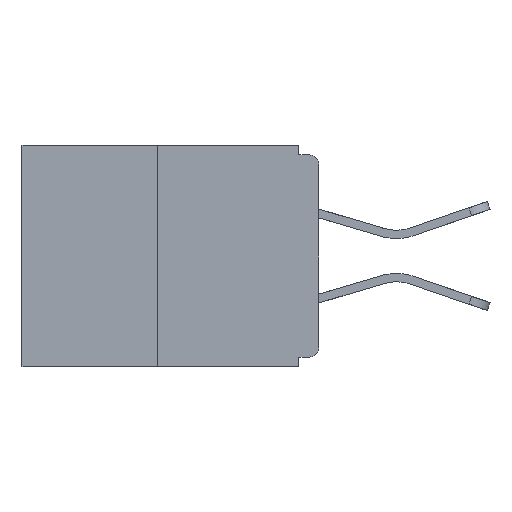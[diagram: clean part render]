
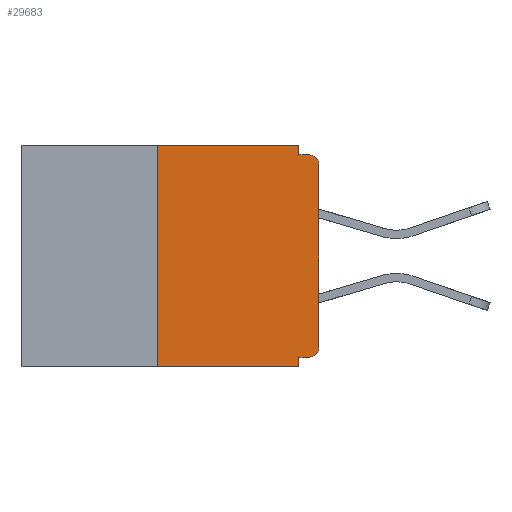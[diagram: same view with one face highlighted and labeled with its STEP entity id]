
A CAD part, left-side view. The second image highlights one B-rep face of the part: STEP entity #29683.
In plain terms, the highlighted planar face has unit normal (-1, 0, 0).
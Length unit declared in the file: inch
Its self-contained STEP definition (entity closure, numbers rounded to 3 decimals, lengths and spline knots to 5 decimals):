
#731 = VECTOR ( 'NONE', #14783, 39.37008 ) ;
#1760 = VECTOR ( 'NONE', #10039, 39.37008 ) ;
#2047 = CIRCLE ( 'NONE', #9286, 0.015 ) ;
#2706 = ORIENTED_EDGE ( 'NONE', *, *, #6965, .F. ) ;
#2714 = ORIENTED_EDGE ( 'NONE', *, *, #26949, .F. ) ;
#3550 = CARTESIAN_POINT ( 'NONE',  ( 0., 0.015, -0.328 ) ) ;
#3679 = VERTEX_POINT ( 'NONE', #21947 ) ;
#3745 = CARTESIAN_POINT ( 'NONE',  ( 0., 0.015, -0.03 ) ) ;
#3855 = DIRECTION ( 'NONE',  ( 0., 0., -1. ) ) ;
#4433 = LINE ( 'NONE', #21259, #26086 ) ;
#4735 = FACE_OUTER_BOUND ( 'NONE', #29015, .T. ) ;
#5065 = ORIENTED_EDGE ( 'NONE', *, *, #28277, .T. ) ;
#5213 = CARTESIAN_POINT ( 'NONE',  ( 0., 0., 0. ) ) ;
#5677 = DIRECTION ( 'NONE',  ( -1., 0., 0. ) ) ;
#5901 = ORIENTED_EDGE ( 'NONE', *, *, #29616, .T. ) ;
#6394 = CARTESIAN_POINT ( 'NONE',  ( 0., 0.031, -0.015 ) ) ;
#6450 = DIRECTION ( 'NONE',  ( 0., 0., -1. ) ) ;
#6664 = CARTESIAN_POINT ( 'NONE',  ( 0., 0., -0.03 ) ) ;
#6965 = EDGE_CURVE ( 'NONE', #22255, #7454, #16489, .T. ) ;
#7068 = VERTEX_POINT ( 'NONE', #9651 ) ;
#7406 = CARTESIAN_POINT ( 'NONE',  ( 0., 0., -0.328 ) ) ;
#7454 = VERTEX_POINT ( 'NONE', #6394 ) ;
#7911 = VERTEX_POINT ( 'NONE', #6664 ) ;
#8894 = CARTESIAN_POINT ( 'NONE',  ( 0., 0.46, -0.343 ) ) ;
#9176 = VECTOR ( 'NONE', #12169, 39.37008 ) ;
#9286 = AXIS2_PLACEMENT_3D ( 'NONE', #3745, #18150, #3855 ) ;
#9651 = CARTESIAN_POINT ( 'NONE',  ( 0., 0., -0.313 ) ) ;
#10039 = DIRECTION ( 'NONE',  ( 0., 0., 1. ) ) ;
#10164 = VECTOR ( 'NONE', #16411, 39.37008 ) ;
#10218 = VERTEX_POINT ( 'NONE', #18093 ) ;
#10365 = CARTESIAN_POINT ( 'NONE',  ( 0., 0.015, -0.313 ) ) ;
#10588 = LINE ( 'NONE', #8894, #20694 ) ;
#10612 = DIRECTION ( 'NONE',  ( 0., 0., -1. ) ) ;
#12142 = ORIENTED_EDGE ( 'NONE', *, *, #27635, .F. ) ;
#12169 = DIRECTION ( 'NONE',  ( 0., 1., 0. ) ) ;
#13222 = CARTESIAN_POINT ( 'NONE',  ( 0., 0.031, -0.343 ) ) ;
#13822 = EDGE_CURVE ( 'NONE', #26939, #7068, #23405, .T. ) ;
#14033 = CARTESIAN_POINT ( 'NONE',  ( 0., 0.031, -0.328 ) ) ;
#14430 = LINE ( 'NONE', #5213, #1760 ) ;
#14516 = VERTEX_POINT ( 'NONE', #14033 ) ;
#14783 = DIRECTION ( 'NONE',  ( 0., -1., 0. ) ) ;
#15462 = AXIS2_PLACEMENT_3D ( 'NONE', #10365, #5677, #22162 ) ;
#16190 = EDGE_CURVE ( 'NONE', #7911, #3679, #2047, .T. ) ;
#16411 = DIRECTION ( 'NONE',  ( 0., 0., -1. ) ) ;
#16489 = LINE ( 'NONE', #16616, #10164 ) ;
#16616 = CARTESIAN_POINT ( 'NONE',  ( 0., 0.031, 0. ) ) ;
#17787 = VECTOR ( 'NONE', #10612, 39.37008 ) ;
#18093 = CARTESIAN_POINT ( 'NONE',  ( 0., 0.25, 0. ) ) ;
#18150 = DIRECTION ( 'NONE',  ( -1., 0., 0. ) ) ;
#18201 = ORIENTED_EDGE ( 'NONE', *, *, #24262, .F. ) ;
#18871 = CARTESIAN_POINT ( 'NONE',  ( 0., 0.25, -0.343 ) ) ;
#18930 = ORIENTED_EDGE ( 'NONE', *, *, #16190, .T. ) ;
#18976 = DIRECTION ( 'NONE',  ( 0., -1., 0. ) ) ;
#19293 = VERTEX_POINT ( 'NONE', #13222 ) ;
#19565 = ORIENTED_EDGE ( 'NONE', *, *, #13822, .T. ) ;
#20343 = CARTESIAN_POINT ( 'NONE',  ( 0., 0.031, -0.343 ) ) ;
#20694 = VECTOR ( 'NONE', #21111, 39.37008 ) ;
#21021 = EDGE_CURVE ( 'NONE', #14516, #19293, #22283, .T. ) ;
#21111 = DIRECTION ( 'NONE',  ( 0., -1., 0. ) ) ;
#21259 = CARTESIAN_POINT ( 'NONE',  ( 0., 0.25, 0. ) ) ;
#21947 = CARTESIAN_POINT ( 'NONE',  ( 0., 0.015, -0.015 ) ) ;
#22109 = CARTESIAN_POINT ( 'NONE',  ( 0., 0., -0.015 ) ) ;
#22162 = DIRECTION ( 'NONE',  ( 0., 0., -1. ) ) ;
#22255 = VERTEX_POINT ( 'NONE', #22966 ) ;
#22283 = LINE ( 'NONE', #20343, #17787 ) ;
#22966 = CARTESIAN_POINT ( 'NONE',  ( 0., 0.031, 0. ) ) ;
#22975 = PLANE ( 'NONE',  #29574 ) ;
#23405 = CIRCLE ( 'NONE', #15462, 0.015 ) ;
#23716 = VECTOR ( 'NONE', #18976, 39.37008 ) ;
#24262 = EDGE_CURVE ( 'NONE', #7454, #3679, #26142, .T. ) ;
#24696 = EDGE_CURVE ( 'NONE', #27689, #10218, #4433, .T. ) ;
#25203 = LINE ( 'NONE', #30383, #23716 ) ;
#25345 = CARTESIAN_POINT ( 'NONE',  ( 0., 0.46, 0. ) ) ;
#25649 = DIRECTION ( 'NONE',  ( 1., 0., 0. ) ) ;
#26086 = VECTOR ( 'NONE', #28238, 39.37008 ) ;
#26142 = LINE ( 'NONE', #22109, #731 ) ;
#26939 = VERTEX_POINT ( 'NONE', #3550 ) ;
#26949 = EDGE_CURVE ( 'NONE', #26939, #14516, #28229, .T. ) ;
#27635 = EDGE_CURVE ( 'NONE', #10218, #22255, #25203, .T. ) ;
#27689 = VERTEX_POINT ( 'NONE', #18871 ) ;
#28229 = LINE ( 'NONE', #7406, #9176 ) ;
#28238 = DIRECTION ( 'NONE',  ( 0., 0., 1. ) ) ;
#28277 = EDGE_CURVE ( 'NONE', #27689, #19293, #10588, .T. ) ;
#29015 = EDGE_LOOP ( 'NONE', ( #12142, #30234, #5065, #30387, #2714, #19565, #5901, #18930, #18201, #2706 ) ) ;
#29574 = AXIS2_PLACEMENT_3D ( 'NONE', #25345, #25649, #6450 ) ;
#29616 = EDGE_CURVE ( 'NONE', #7068, #7911, #14430, .T. ) ;
#29683 = ADVANCED_FACE ( 'NONE', ( #4735 ), #22975, .F. ) ;
#30234 = ORIENTED_EDGE ( 'NONE', *, *, #24696, .F. ) ;
#30383 = CARTESIAN_POINT ( 'NONE',  ( 0., 0.46, 0. ) ) ;
#30387 = ORIENTED_EDGE ( 'NONE', *, *, #21021, .F. ) ;
